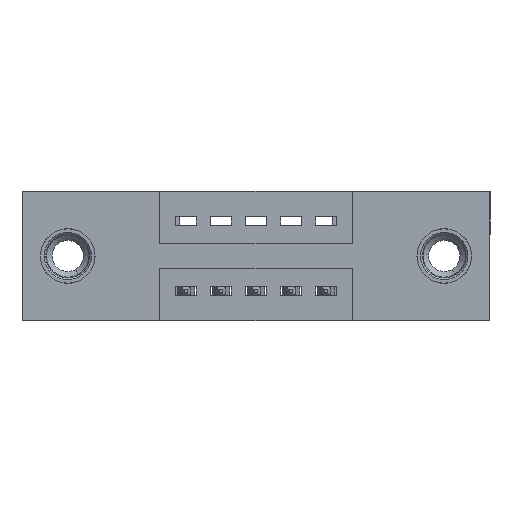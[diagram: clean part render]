
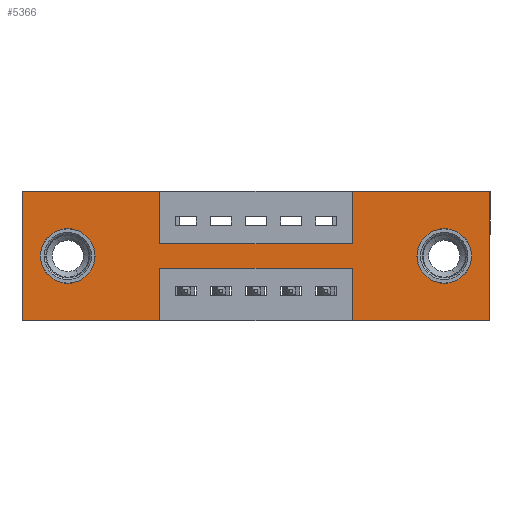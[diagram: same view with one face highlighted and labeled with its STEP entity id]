
A CAD part, front view. The second image highlights one B-rep face of the part: STEP entity #5366.
In plain terms, the highlighted planar face has unit normal (0, -1, 0).
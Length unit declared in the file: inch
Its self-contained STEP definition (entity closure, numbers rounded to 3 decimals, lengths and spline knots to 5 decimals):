
#35 = CARTESIAN_POINT ( 'NONE',  ( 0.9425, 0., -0.15 ) ) ;
#55 = LINE ( 'NONE', #6821, #10474 ) ;
#256 = CIRCLE ( 'NONE', #8845, 0.078 ) ;
#350 = DIRECTION ( 'NONE',  ( 1., 0., 0. ) ) ;
#458 = CARTESIAN_POINT ( 'NONE',  ( 0.13, 0., -0.107 ) ) ;
#518 = AXIS2_PLACEMENT_3D ( 'NONE', #2571, #5995, #6798 ) ;
#974 = CARTESIAN_POINT ( 'NONE',  ( 1.205, 0., -0.185 ) ) ;
#984 = LINE ( 'NONE', #6089, #10886 ) ;
#998 = DIRECTION ( 'NONE',  ( 1., 0., 0. ) ) ;
#1001 = EDGE_CURVE ( 'NONE', #5294, #1051, #7973, .T. ) ;
#1051 = VERTEX_POINT ( 'NONE', #9365 ) ;
#1093 = LINE ( 'NONE', #6667, #1368 ) ;
#1142 = CARTESIAN_POINT ( 'NONE',  ( 0.13, 0., -0.185 ) ) ;
#1272 = EDGE_CURVE ( 'NONE', #8696, #7837, #984, .T. ) ;
#1338 = DIRECTION ( 'NONE',  ( 0., 0., -1. ) ) ;
#1368 = VECTOR ( 'NONE', #3324, 39.37008 ) ;
#1548 = CARTESIAN_POINT ( 'NONE',  ( 1.335, 0., -0.37 ) ) ;
#1551 = EDGE_CURVE ( 'NONE', #1639, #7312, #6920, .T. ) ;
#1603 = CARTESIAN_POINT ( 'NONE',  ( 0., 0., 0. ) ) ;
#1630 = CARTESIAN_POINT ( 'NONE',  ( 0.9425, 0., 0. ) ) ;
#1639 = VERTEX_POINT ( 'NONE', #4323 ) ;
#1941 = DIRECTION ( 'NONE',  ( 0., 0., 1. ) ) ;
#2032 = VECTOR ( 'NONE', #10916, 39.37008 ) ;
#2063 = FACE_BOUND ( 'NONE', #5536, .T. ) ;
#2153 = DIRECTION ( 'NONE',  ( 0., 0., -1. ) ) ;
#2173 = VECTOR ( 'NONE', #350, 39.37008 ) ;
#2471 = EDGE_CURVE ( 'NONE', #10042, #6323, #3088, .T. ) ;
#2506 = EDGE_CURVE ( 'NONE', #7312, #8696, #5047, .T. ) ;
#2561 = LINE ( 'NONE', #9582, #5452 ) ;
#2571 = CARTESIAN_POINT ( 'NONE',  ( 1.205, 0., -0.185 ) ) ;
#2700 = CARTESIAN_POINT ( 'NONE',  ( 0.13, 0., -0.185 ) ) ;
#2701 = DIRECTION ( 'NONE',  ( 0., 1., 0. ) ) ;
#2752 = EDGE_CURVE ( 'NONE', #1051, #5991, #8867, .T. ) ;
#2780 = ORIENTED_EDGE ( 'NONE', *, *, #2471, .F. ) ;
#2794 = CARTESIAN_POINT ( 'NONE',  ( 1.205, 0., -0.107 ) ) ;
#2877 = ORIENTED_EDGE ( 'NONE', *, *, #6990, .F. ) ;
#2922 = CARTESIAN_POINT ( 'NONE',  ( 0., 0., 0. ) ) ;
#2934 = DIRECTION ( 'NONE',  ( 0., -1., 0. ) ) ;
#3088 = LINE ( 'NONE', #7894, #9540 ) ;
#3321 = ORIENTED_EDGE ( 'NONE', *, *, #4836, .T. ) ;
#3324 = DIRECTION ( 'NONE',  ( -1., 0., 0. ) ) ;
#3337 = VERTEX_POINT ( 'NONE', #7490 ) ;
#3493 = VERTEX_POINT ( 'NONE', #1630 ) ;
#3575 = ORIENTED_EDGE ( 'NONE', *, *, #6532, .F. ) ;
#3744 = EDGE_CURVE ( 'NONE', #6307, #3337, #256, .T. ) ;
#3763 = CARTESIAN_POINT ( 'NONE',  ( 0.3925, 0., -0.15 ) ) ;
#3838 = PLANE ( 'NONE',  #7022 ) ;
#3939 = CIRCLE ( 'NONE', #9996, 0.078 ) ;
#4132 = ORIENTED_EDGE ( 'NONE', *, *, #7343, .F. ) ;
#4158 = EDGE_LOOP ( 'NONE', ( #7504, #2877, #3575, #4132, #2780, #7378, #6530, #7101, #5650, #6004, #6194, #4365 ) ) ;
#4259 = EDGE_CURVE ( 'NONE', #7531, #9168, #3939, .T. ) ;
#4286 = VECTOR ( 'NONE', #6278, 39.37008 ) ;
#4315 = DIRECTION ( 'NONE',  ( 0., 0., -1. ) ) ;
#4323 = CARTESIAN_POINT ( 'NONE',  ( 0., 0., 0. ) ) ;
#4365 = ORIENTED_EDGE ( 'NONE', *, *, #2752, .F. ) ;
#4566 = CARTESIAN_POINT ( 'NONE',  ( 0.9425, 0., -0.22 ) ) ;
#4623 = CARTESIAN_POINT ( 'NONE',  ( 0.3925, 0., 0. ) ) ;
#4642 = ORIENTED_EDGE ( 'NONE', *, *, #3744, .T. ) ;
#4836 = EDGE_CURVE ( 'NONE', #9168, #7531, #6547, .T. ) ;
#4940 = CARTESIAN_POINT ( 'NONE',  ( 0.3925, 0., 0. ) ) ;
#5047 = LINE ( 'NONE', #4623, #9943 ) ;
#5107 = FACE_BOUND ( 'NONE', #7400, .T. ) ;
#5193 = DIRECTION ( 'NONE',  ( -1., 0., 0. ) ) ;
#5294 = VERTEX_POINT ( 'NONE', #8775 ) ;
#5309 = DIRECTION ( 'NONE',  ( 0., 1., 0. ) ) ;
#5342 = DIRECTION ( 'NONE',  ( 0., 0., 1. ) ) ;
#5366 = ADVANCED_FACE ( 'NONE', ( #5107, #2063, #9189 ), #3838, .T. ) ;
#5452 = VECTOR ( 'NONE', #5193, 39.37008 ) ;
#5536 = EDGE_LOOP ( 'NONE', ( #4642, #9256 ) ) ;
#5608 = CARTESIAN_POINT ( 'NONE',  ( 1.205, 0., -0.263 ) ) ;
#5650 = ORIENTED_EDGE ( 'NONE', *, *, #2506, .F. ) ;
#5991 = VERTEX_POINT ( 'NONE', #6115 ) ;
#5995 = DIRECTION ( 'NONE',  ( 0., 1., 0. ) ) ;
#6004 = ORIENTED_EDGE ( 'NONE', *, *, #1551, .F. ) ;
#6016 = CARTESIAN_POINT ( 'NONE',  ( 0.9425, 0., 0. ) ) ;
#6089 = CARTESIAN_POINT ( 'NONE',  ( 0.3925, 0., -0.15 ) ) ;
#6115 = CARTESIAN_POINT ( 'NONE',  ( 0., 0., -0.37 ) ) ;
#6149 = EDGE_CURVE ( 'NONE', #3493, #10042, #6787, .T. ) ;
#6194 = ORIENTED_EDGE ( 'NONE', *, *, #9864, .F. ) ;
#6210 = CARTESIAN_POINT ( 'NONE',  ( 0., 0., 0. ) ) ;
#6278 = DIRECTION ( 'NONE',  ( 0., 0., 1. ) ) ;
#6282 = VERTEX_POINT ( 'NONE', #9982 ) ;
#6307 = VERTEX_POINT ( 'NONE', #458 ) ;
#6311 = DIRECTION ( 'NONE',  ( 1., 0., 0. ) ) ;
#6323 = VERTEX_POINT ( 'NONE', #1548 ) ;
#6369 = CARTESIAN_POINT ( 'NONE',  ( 0., 0., -0.37 ) ) ;
#6530 = ORIENTED_EDGE ( 'NONE', *, *, #9315, .F. ) ;
#6532 = EDGE_CURVE ( 'NONE', #6282, #9790, #55, .T. ) ;
#6547 = CIRCLE ( 'NONE', #518, 0.078 ) ;
#6667 = CARTESIAN_POINT ( 'NONE',  ( 0., 0., -0.37 ) ) ;
#6766 = ORIENTED_EDGE ( 'NONE', *, *, #4259, .T. ) ;
#6787 = LINE ( 'NONE', #6210, #10486 ) ;
#6798 = DIRECTION ( 'NONE',  ( 0., 0., -1. ) ) ;
#6821 = CARTESIAN_POINT ( 'NONE',  ( 0.9425, 0., -0.37 ) ) ;
#6867 = DIRECTION ( 'NONE',  ( 0., 1., 0. ) ) ;
#6920 = LINE ( 'NONE', #1603, #2173 ) ;
#6990 = EDGE_CURVE ( 'NONE', #9790, #5294, #2561, .T. ) ;
#7022 = AXIS2_PLACEMENT_3D ( 'NONE', #6369, #2934, #1338 ) ;
#7101 = ORIENTED_EDGE ( 'NONE', *, *, #1272, .F. ) ;
#7164 = DIRECTION ( 'NONE',  ( 0., 0., -1. ) ) ;
#7312 = VERTEX_POINT ( 'NONE', #4940 ) ;
#7343 = EDGE_CURVE ( 'NONE', #6323, #6282, #1093, .T. ) ;
#7378 = ORIENTED_EDGE ( 'NONE', *, *, #6149, .F. ) ;
#7400 = EDGE_LOOP ( 'NONE', ( #6766, #3321 ) ) ;
#7490 = CARTESIAN_POINT ( 'NONE',  ( 0.13, 0., -0.263 ) ) ;
#7504 = ORIENTED_EDGE ( 'NONE', *, *, #1001, .F. ) ;
#7531 = VERTEX_POINT ( 'NONE', #2794 ) ;
#7837 = VERTEX_POINT ( 'NONE', #35 ) ;
#7894 = CARTESIAN_POINT ( 'NONE',  ( 1.335, 0., 0. ) ) ;
#7973 = LINE ( 'NONE', #8391, #2032 ) ;
#8245 = AXIS2_PLACEMENT_3D ( 'NONE', #2700, #5309, #1941 ) ;
#8391 = CARTESIAN_POINT ( 'NONE',  ( 0.3925, 0., -0.37 ) ) ;
#8696 = VERTEX_POINT ( 'NONE', #3763 ) ;
#8754 = CARTESIAN_POINT ( 'NONE',  ( 0., 0., -0.37 ) ) ;
#8775 = CARTESIAN_POINT ( 'NONE',  ( 0.3925, 0., -0.22 ) ) ;
#8789 = DIRECTION ( 'NONE',  ( -1., 0., 0. ) ) ;
#8845 = AXIS2_PLACEMENT_3D ( 'NONE', #1142, #2701, #9449 ) ;
#8867 = LINE ( 'NONE', #8754, #10842 ) ;
#9168 = VERTEX_POINT ( 'NONE', #5608 ) ;
#9189 = FACE_OUTER_BOUND ( 'NONE', #4158, .T. ) ;
#9256 = ORIENTED_EDGE ( 'NONE', *, *, #9388, .T. ) ;
#9315 = EDGE_CURVE ( 'NONE', #7837, #3493, #10004, .T. ) ;
#9365 = CARTESIAN_POINT ( 'NONE',  ( 0.3925, 0., -0.37 ) ) ;
#9388 = EDGE_CURVE ( 'NONE', #3337, #6307, #10784, .T. ) ;
#9413 = DIRECTION ( 'NONE',  ( 0., 0., 1. ) ) ;
#9449 = DIRECTION ( 'NONE',  ( 0., 0., 1. ) ) ;
#9540 = VECTOR ( 'NONE', #7164, 39.37008 ) ;
#9582 = CARTESIAN_POINT ( 'NONE',  ( 0.3925, 0., -0.22 ) ) ;
#9737 = VECTOR ( 'NONE', #5342, 39.37008 ) ;
#9790 = VERTEX_POINT ( 'NONE', #4566 ) ;
#9864 = EDGE_CURVE ( 'NONE', #5991, #1639, #10109, .T. ) ;
#9943 = VECTOR ( 'NONE', #2153, 39.37008 ) ;
#9982 = CARTESIAN_POINT ( 'NONE',  ( 0.9425, 0., -0.37 ) ) ;
#9996 = AXIS2_PLACEMENT_3D ( 'NONE', #974, #6867, #4315 ) ;
#10004 = LINE ( 'NONE', #6016, #9737 ) ;
#10042 = VERTEX_POINT ( 'NONE', #10297 ) ;
#10109 = LINE ( 'NONE', #2922, #4286 ) ;
#10297 = CARTESIAN_POINT ( 'NONE',  ( 1.335, 0., 0. ) ) ;
#10474 = VECTOR ( 'NONE', #9413, 39.37008 ) ;
#10486 = VECTOR ( 'NONE', #6311, 39.37008 ) ;
#10784 = CIRCLE ( 'NONE', #8245, 0.078 ) ;
#10842 = VECTOR ( 'NONE', #8789, 39.37008 ) ;
#10886 = VECTOR ( 'NONE', #998, 39.37008 ) ;
#10916 = DIRECTION ( 'NONE',  ( 0., 0., -1. ) ) ;
